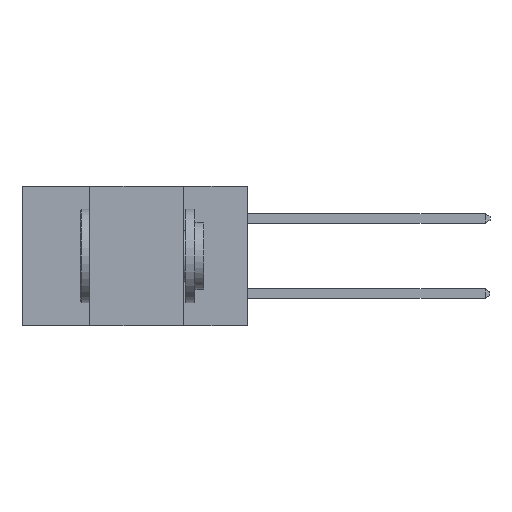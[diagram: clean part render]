
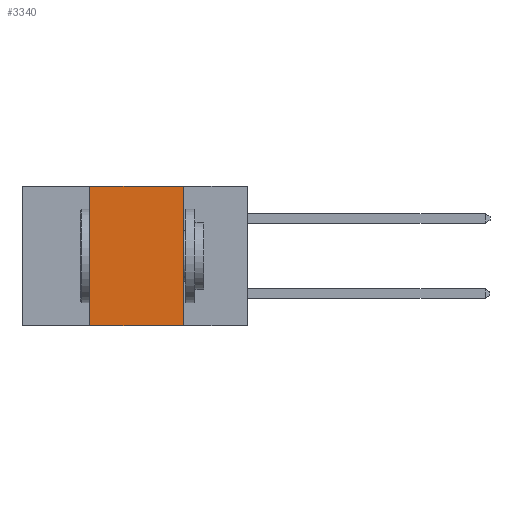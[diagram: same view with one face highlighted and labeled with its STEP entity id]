
A CAD part, left-side view. The second image highlights one B-rep face of the part: STEP entity #3340.
In plain terms, the highlighted planar face has unit normal (-1, 0, 0).
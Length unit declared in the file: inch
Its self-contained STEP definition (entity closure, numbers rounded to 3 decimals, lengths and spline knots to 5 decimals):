
#991 = EDGE_LOOP ( 'NONE', ( #14321, #11988, #4377, #10830 ) ) ;
#1129 = CARTESIAN_POINT ( 'NONE',  ( 0., 0.6, -0.37 ) ) ;
#2288 = CARTESIAN_POINT ( 'NONE',  ( 0., 0.6, 0. ) ) ;
#2904 = LINE ( 'NONE', #2288, #16008 ) ;
#3006 = LINE ( 'NONE', #7742, #12801 ) ;
#3340 = ADVANCED_FACE ( 'NONE', ( #10663 ), #7335, .F. ) ;
#4204 = CARTESIAN_POINT ( 'NONE',  ( 0., 0.17, 0. ) ) ;
#4377 = ORIENTED_EDGE ( 'NONE', *, *, #15344, .F. ) ;
#4528 = CARTESIAN_POINT ( 'NONE',  ( 0., 0.42, 0. ) ) ;
#4838 = DIRECTION ( 'NONE',  ( 0., 0., -1. ) ) ;
#5431 = EDGE_CURVE ( 'NONE', #5511, #8131, #2904, .T. ) ;
#5511 = VERTEX_POINT ( 'NONE', #4528 ) ;
#5515 = CARTESIAN_POINT ( 'NONE',  ( 0., 0.42, 0. ) ) ;
#6686 = VECTOR ( 'NONE', #9387, 39.37008 ) ;
#7335 = PLANE ( 'NONE',  #16263 ) ;
#7742 = CARTESIAN_POINT ( 'NONE',  ( 0., 0.17, 0. ) ) ;
#8131 = VERTEX_POINT ( 'NONE', #4204 ) ;
#8712 = CARTESIAN_POINT ( 'NONE',  ( 0., 0.6, 0. ) ) ;
#9387 = DIRECTION ( 'NONE',  ( 0., 0., 1. ) ) ;
#9498 = VERTEX_POINT ( 'NONE', #10661 ) ;
#9957 = EDGE_CURVE ( 'NONE', #15780, #9498, #11005, .T. ) ;
#10191 = DIRECTION ( 'NONE',  ( 1., 0., 0. ) ) ;
#10220 = DIRECTION ( 'NONE',  ( 0., 0., -1. ) ) ;
#10467 = LINE ( 'NONE', #5515, #6686 ) ;
#10661 = CARTESIAN_POINT ( 'NONE',  ( 0., 0.17, -0.37 ) ) ;
#10663 = FACE_OUTER_BOUND ( 'NONE', #991, .T. ) ;
#10830 = ORIENTED_EDGE ( 'NONE', *, *, #9957, .T. ) ;
#11005 = LINE ( 'NONE', #1129, #13947 ) ;
#11988 = ORIENTED_EDGE ( 'NONE', *, *, #5431, .F. ) ;
#12801 = VECTOR ( 'NONE', #10220, 39.37008 ) ;
#12937 = DIRECTION ( 'NONE',  ( 0., -1., 0. ) ) ;
#13947 = VECTOR ( 'NONE', #16524, 39.37008 ) ;
#13972 = CARTESIAN_POINT ( 'NONE',  ( 0., 0.42, -0.37 ) ) ;
#14321 = ORIENTED_EDGE ( 'NONE', *, *, #15133, .F. ) ;
#15133 = EDGE_CURVE ( 'NONE', #8131, #9498, #3006, .T. ) ;
#15344 = EDGE_CURVE ( 'NONE', #15780, #5511, #10467, .T. ) ;
#15780 = VERTEX_POINT ( 'NONE', #13972 ) ;
#16008 = VECTOR ( 'NONE', #12937, 39.37008 ) ;
#16263 = AXIS2_PLACEMENT_3D ( 'NONE', #8712, #10191, #4838 ) ;
#16524 = DIRECTION ( 'NONE',  ( 0., -1., 0. ) ) ;
